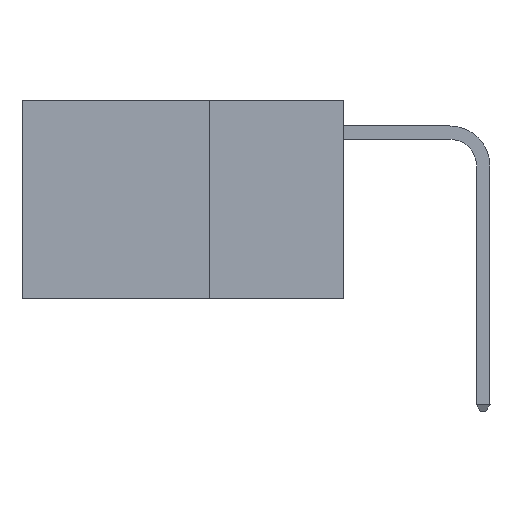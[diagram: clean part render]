
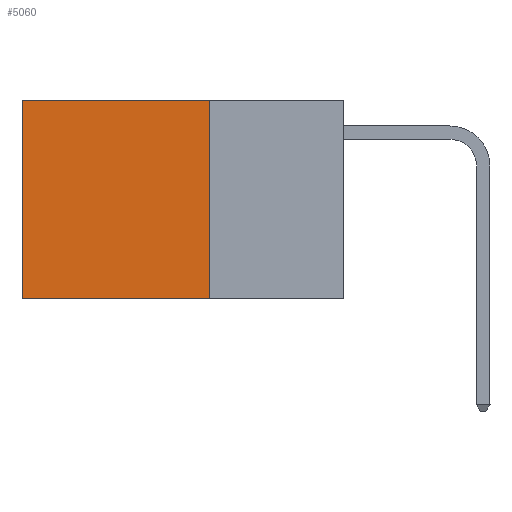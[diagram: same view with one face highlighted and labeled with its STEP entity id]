
A CAD part, left-side view. The second image highlights one B-rep face of the part: STEP entity #5060.
In plain terms, the highlighted planar face has unit normal (-1, 0, 0).
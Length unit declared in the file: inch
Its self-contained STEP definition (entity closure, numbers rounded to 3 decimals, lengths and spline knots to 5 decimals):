
#114 = EDGE_LOOP ( 'NONE', ( #7202, #15266, #2221, #1083 ) ) ;
#355 = LINE ( 'NONE', #9185, #2983 ) ;
#400 = VERTEX_POINT ( 'NONE', #15518 ) ;
#1026 = DIRECTION ( 'NONE',  ( 0., 0., -1. ) ) ;
#1083 = ORIENTED_EDGE ( 'NONE', *, *, #9839, .T. ) ;
#1228 = EDGE_CURVE ( 'NONE', #9328, #7189, #10392, .T. ) ;
#1336 = AXIS2_PLACEMENT_3D ( 'NONE', #2274, #8627, #1026 ) ;
#2221 = ORIENTED_EDGE ( 'NONE', *, *, #9418, .F. ) ;
#2274 = CARTESIAN_POINT ( 'NONE',  ( 0.2625, 0.25, 0. ) ) ;
#2983 = VECTOR ( 'NONE', #6740, 39.37008 ) ;
#3753 = VECTOR ( 'NONE', #10257, 39.37008 ) ;
#4651 = DIRECTION ( 'NONE',  ( 0., 0., -1. ) ) ;
#4679 = CARTESIAN_POINT ( 'NONE',  ( 0.2625, 0.6, 0. ) ) ;
#5060 = ADVANCED_FACE ( 'NONE', ( #5615 ), #15927, .F. ) ;
#5322 = CARTESIAN_POINT ( 'NONE',  ( 0.2625, 0.25, 0. ) ) ;
#5615 = FACE_OUTER_BOUND ( 'NONE', #114, .T. ) ;
#5967 = DIRECTION ( 'NONE',  ( 0., 0., -1. ) ) ;
#6740 = DIRECTION ( 'NONE',  ( 0., 1., 0. ) ) ;
#6772 = EDGE_CURVE ( 'NONE', #400, #7189, #11088, .T. ) ;
#6773 = VECTOR ( 'NONE', #4651, 39.37008 ) ;
#7189 = VERTEX_POINT ( 'NONE', #8017 ) ;
#7202 = ORIENTED_EDGE ( 'NONE', *, *, #6772, .T. ) ;
#7816 = VECTOR ( 'NONE', #5967, 39.37008 ) ;
#8017 = CARTESIAN_POINT ( 'NONE',  ( 0.2625, 0.6, -0.37 ) ) ;
#8627 = DIRECTION ( 'NONE',  ( 1., 0., 0. ) ) ;
#9185 = CARTESIAN_POINT ( 'NONE',  ( 0.2625, 0.25, 0. ) ) ;
#9328 = VERTEX_POINT ( 'NONE', #15552 ) ;
#9418 = EDGE_CURVE ( 'NONE', #12072, #9328, #12550, .T. ) ;
#9839 = EDGE_CURVE ( 'NONE', #12072, #400, #355, .T. ) ;
#10257 = DIRECTION ( 'NONE',  ( 0., 1., 0. ) ) ;
#10392 = LINE ( 'NONE', #10474, #3753 ) ;
#10474 = CARTESIAN_POINT ( 'NONE',  ( 0.2625, 0.25, -0.37 ) ) ;
#11088 = LINE ( 'NONE', #4679, #7816 ) ;
#12072 = VERTEX_POINT ( 'NONE', #5322 ) ;
#12088 = CARTESIAN_POINT ( 'NONE',  ( 0.2625, 0.25, 0. ) ) ;
#12550 = LINE ( 'NONE', #12088, #6773 ) ;
#15266 = ORIENTED_EDGE ( 'NONE', *, *, #1228, .F. ) ;
#15518 = CARTESIAN_POINT ( 'NONE',  ( 0.2625, 0.6, 0. ) ) ;
#15552 = CARTESIAN_POINT ( 'NONE',  ( 0.2625, 0.25, -0.37 ) ) ;
#15927 = PLANE ( 'NONE',  #1336 ) ;
